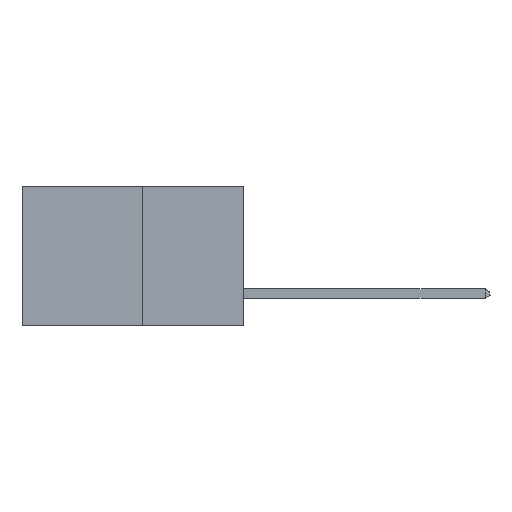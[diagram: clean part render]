
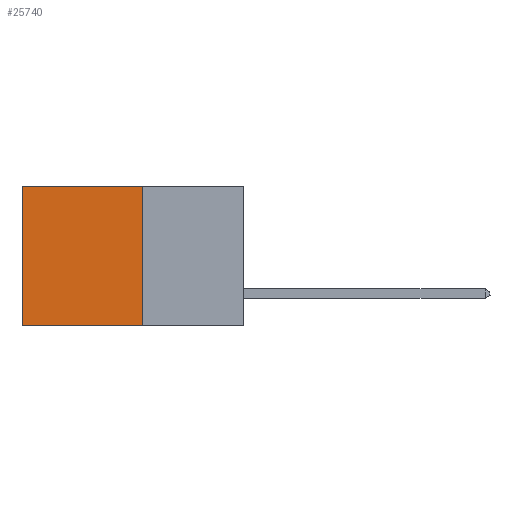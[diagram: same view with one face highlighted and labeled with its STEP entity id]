
A CAD part, left-side view. The second image highlights one B-rep face of the part: STEP entity #25740.
In plain terms, the highlighted planar face has unit normal (-1, 0, 0).
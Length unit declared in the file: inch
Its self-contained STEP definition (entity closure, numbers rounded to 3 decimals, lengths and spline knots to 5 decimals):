
#603 = DIRECTION ( 'NONE',  ( 0., 1., 0. ) ) ;
#1386 = DIRECTION ( 'NONE',  ( 0., 0., -1. ) ) ;
#1907 = DIRECTION ( 'NONE',  ( 0., 1., 0. ) ) ;
#4700 = VECTOR ( 'NONE', #1386, 39.37008 ) ;
#5970 = CARTESIAN_POINT ( 'NONE',  ( 0.277, 0.27, 0. ) ) ;
#6004 = ORIENTED_EDGE ( 'NONE', *, *, #20721, .F. ) ;
#6112 = VERTEX_POINT ( 'NONE', #7805 ) ;
#6842 = ORIENTED_EDGE ( 'NONE', *, *, #27963, .F. ) ;
#7342 = FACE_OUTER_BOUND ( 'NONE', #12348, .T. ) ;
#7805 = CARTESIAN_POINT ( 'NONE',  ( 0.277, 0.59, -0.37 ) ) ;
#7954 = CARTESIAN_POINT ( 'NONE',  ( 0.277, 0.59, -0.37 ) ) ;
#8011 = AXIS2_PLACEMENT_3D ( 'NONE', #30925, #33468, #18000 ) ;
#9283 = VECTOR ( 'NONE', #603, 39.37008 ) ;
#9346 = VECTOR ( 'NONE', #1907, 39.37008 ) ;
#12348 = EDGE_LOOP ( 'NONE', ( #32167, #6004, #6842, #28957 ) ) ;
#12834 = PLANE ( 'NONE',  #8011 ) ;
#14740 = CARTESIAN_POINT ( 'NONE',  ( 0.277, 0.27, -0.37 ) ) ;
#15215 = VERTEX_POINT ( 'NONE', #14740 ) ;
#15873 = EDGE_CURVE ( 'NONE', #18544, #22533, #30036, .T. ) ;
#16170 = LINE ( 'NONE', #29069, #9283 ) ;
#17224 = VECTOR ( 'NONE', #20831, 39.37008 ) ;
#18000 = DIRECTION ( 'NONE',  ( 0., 0., -1. ) ) ;
#18544 = VERTEX_POINT ( 'NONE', #5970 ) ;
#20721 = EDGE_CURVE ( 'NONE', #15215, #6112, #16170, .T. ) ;
#20831 = DIRECTION ( 'NONE',  ( 0., 0., -1. ) ) ;
#22533 = VERTEX_POINT ( 'NONE', #22801 ) ;
#22801 = CARTESIAN_POINT ( 'NONE',  ( 0.277, 0.59, 0. ) ) ;
#25369 = LINE ( 'NONE', #32381, #4700 ) ;
#25740 = ADVANCED_FACE ( 'NONE', ( #7342 ), #12834, .F. ) ;
#27963 = EDGE_CURVE ( 'NONE', #18544, #15215, #25369, .T. ) ;
#28182 = EDGE_CURVE ( 'NONE', #22533, #6112, #31018, .T. ) ;
#28957 = ORIENTED_EDGE ( 'NONE', *, *, #15873, .T. ) ;
#29069 = CARTESIAN_POINT ( 'NONE',  ( 0.277, 0.27, -0.37 ) ) ;
#30036 = LINE ( 'NONE', #32870, #9346 ) ;
#30925 = CARTESIAN_POINT ( 'NONE',  ( 0.277, 0.27, -0.37 ) ) ;
#31018 = LINE ( 'NONE', #7954, #17224 ) ;
#32167 = ORIENTED_EDGE ( 'NONE', *, *, #28182, .T. ) ;
#32381 = CARTESIAN_POINT ( 'NONE',  ( 0.277, 0.27, -0.37 ) ) ;
#32870 = CARTESIAN_POINT ( 'NONE',  ( 0.277, 0.27, 0. ) ) ;
#33468 = DIRECTION ( 'NONE',  ( 1., 0., 0. ) ) ;
